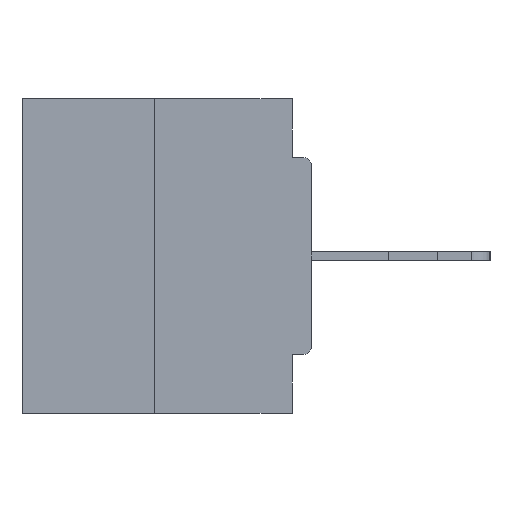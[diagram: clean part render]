
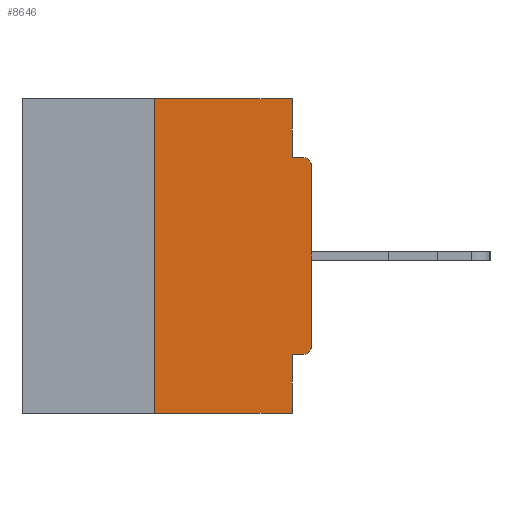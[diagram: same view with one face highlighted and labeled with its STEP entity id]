
A CAD part, left-side view. The second image highlights one B-rep face of the part: STEP entity #8646.
In plain terms, the highlighted planar face has unit normal (-1, 0, 0).
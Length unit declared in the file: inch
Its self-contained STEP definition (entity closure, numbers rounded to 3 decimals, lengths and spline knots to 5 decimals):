
#149 = ORIENTED_EDGE ( 'NONE', *, *, #8234, .F. ) ;
#605 = LINE ( 'NONE', #27355, #24808 ) ;
#615 = LINE ( 'NONE', #12109, #26705 ) ;
#1014 = EDGE_CURVE ( 'NONE', #3477, #11156, #14112, .T. ) ;
#1079 = VERTEX_POINT ( 'NONE', #6250 ) ;
#1119 = EDGE_CURVE ( 'NONE', #1079, #21119, #18806, .T. ) ;
#1353 = VERTEX_POINT ( 'NONE', #11446 ) ;
#1590 = DIRECTION ( 'NONE',  ( 0., 0., -1. ) ) ;
#3269 = CARTESIAN_POINT ( 'NONE',  ( 0., 0.031, 0. ) ) ;
#3477 = VERTEX_POINT ( 'NONE', #12547 ) ;
#3612 = ORIENTED_EDGE ( 'NONE', *, *, #9767, .F. ) ;
#3628 = CARTESIAN_POINT ( 'NONE',  ( 0., 0.015, -0.3915 ) ) ;
#3870 = CARTESIAN_POINT ( 'NONE',  ( 0., 0.031, -0.0935 ) ) ;
#4341 = ORIENTED_EDGE ( 'NONE', *, *, #8951, .T. ) ;
#4351 = ORIENTED_EDGE ( 'NONE', *, *, #15513, .F. ) ;
#4420 = VECTOR ( 'NONE', #23485, 39.37008 ) ;
#4448 = ORIENTED_EDGE ( 'NONE', *, *, #9944, .F. ) ;
#4817 = CARTESIAN_POINT ( 'NONE',  ( 0., 0.25, 0. ) ) ;
#4937 = DIRECTION ( 'NONE',  ( 0., -1., 0. ) ) ;
#5489 = PLANE ( 'NONE',  #23895 ) ;
#6250 = CARTESIAN_POINT ( 'NONE',  ( 0., 0.015, -0.4065 ) ) ;
#6367 = AXIS2_PLACEMENT_3D ( 'NONE', #28479, #19087, #1590 ) ;
#7471 = VERTEX_POINT ( 'NONE', #18476 ) ;
#8234 = EDGE_CURVE ( 'NONE', #21190, #18710, #13362, .T. ) ;
#8646 = ADVANCED_FACE ( 'NONE', ( #23142 ), #5489, .F. ) ;
#8951 = EDGE_CURVE ( 'NONE', #3477, #7471, #615, .T. ) ;
#9069 = CARTESIAN_POINT ( 'NONE',  ( 0., 0.015, -0.0935 ) ) ;
#9613 = VECTOR ( 'NONE', #9849, 39.37008 ) ;
#9767 = EDGE_CURVE ( 'NONE', #1079, #1353, #605, .T. ) ;
#9849 = DIRECTION ( 'NONE',  ( 0., -1., 0. ) ) ;
#9944 = EDGE_CURVE ( 'NONE', #1353, #7471, #24639, .T. ) ;
#9987 = DIRECTION ( 'NONE',  ( 0., 0., -1. ) ) ;
#10577 = CARTESIAN_POINT ( 'NONE',  ( 0., 0., 0. ) ) ;
#11148 = ORIENTED_EDGE ( 'NONE', *, *, #14624, .F. ) ;
#11156 = VERTEX_POINT ( 'NONE', #23710 ) ;
#11260 = DIRECTION ( 'NONE',  ( 0., 1., 0. ) ) ;
#11446 = CARTESIAN_POINT ( 'NONE',  ( 0., 0.031, -0.4065 ) ) ;
#12109 = CARTESIAN_POINT ( 'NONE',  ( 0., 0.46, -0.5 ) ) ;
#12180 = ORIENTED_EDGE ( 'NONE', *, *, #1014, .F. ) ;
#12547 = CARTESIAN_POINT ( 'NONE',  ( 0., 0.25, -0.5 ) ) ;
#13362 = LINE ( 'NONE', #24346, #19172 ) ;
#13501 = DIRECTION ( 'NONE',  ( 0., 0., -1. ) ) ;
#13649 = LINE ( 'NONE', #27414, #9613 ) ;
#14112 = LINE ( 'NONE', #4817, #4420 ) ;
#14342 = EDGE_CURVE ( 'NONE', #26387, #20639, #28772, .T. ) ;
#14620 = AXIS2_PLACEMENT_3D ( 'NONE', #3628, #28487, #23939 ) ;
#14624 = EDGE_CURVE ( 'NONE', #11156, #21190, #13649, .T. ) ;
#15513 = EDGE_CURVE ( 'NONE', #18710, #20639, #16740, .T. ) ;
#16740 = LINE ( 'NONE', #25235, #20365 ) ;
#16809 = EDGE_CURVE ( 'NONE', #21119, #26387, #26370, .T. ) ;
#17094 = VECTOR ( 'NONE', #24431, 39.37008 ) ;
#18476 = CARTESIAN_POINT ( 'NONE',  ( 0., 0.031, -0.5 ) ) ;
#18710 = VERTEX_POINT ( 'NONE', #3870 ) ;
#18806 = CIRCLE ( 'NONE', #14620, 0.015 ) ;
#19087 = DIRECTION ( 'NONE',  ( -1., 0., 0. ) ) ;
#19172 = VECTOR ( 'NONE', #13501, 39.37008 ) ;
#20365 = VECTOR ( 'NONE', #4937, 39.37008 ) ;
#20639 = VERTEX_POINT ( 'NONE', #9069 ) ;
#21119 = VERTEX_POINT ( 'NONE', #26602 ) ;
#21190 = VERTEX_POINT ( 'NONE', #3269 ) ;
#21809 = ORIENTED_EDGE ( 'NONE', *, *, #14342, .T. ) ;
#21879 = ORIENTED_EDGE ( 'NONE', *, *, #16809, .T. ) ;
#22956 = DIRECTION ( 'NONE',  ( 0., -1., 0. ) ) ;
#23142 = FACE_OUTER_BOUND ( 'NONE', #24683, .T. ) ;
#23287 = DIRECTION ( 'NONE',  ( 1., 0., 0. ) ) ;
#23485 = DIRECTION ( 'NONE',  ( 0., 0., 1. ) ) ;
#23710 = CARTESIAN_POINT ( 'NONE',  ( 0., 0.25, 0. ) ) ;
#23895 = AXIS2_PLACEMENT_3D ( 'NONE', #25642, #23287, #9987 ) ;
#23939 = DIRECTION ( 'NONE',  ( 0., 0., -1. ) ) ;
#24284 = CARTESIAN_POINT ( 'NONE',  ( 0., 0., -0.1085 ) ) ;
#24346 = CARTESIAN_POINT ( 'NONE',  ( 0., 0.031, 0. ) ) ;
#24431 = DIRECTION ( 'NONE',  ( 0., 0., 1. ) ) ;
#24639 = LINE ( 'NONE', #26475, #25735 ) ;
#24683 = EDGE_LOOP ( 'NONE', ( #11148, #12180, #4341, #4448, #3612, #26940, #21879, #21809, #4351, #149 ) ) ;
#24808 = VECTOR ( 'NONE', #11260, 39.37008 ) ;
#25235 = CARTESIAN_POINT ( 'NONE',  ( 0., 0., -0.0935 ) ) ;
#25642 = CARTESIAN_POINT ( 'NONE',  ( 0., 0.46, 0. ) ) ;
#25735 = VECTOR ( 'NONE', #26702, 39.37008 ) ;
#26370 = LINE ( 'NONE', #10577, #17094 ) ;
#26387 = VERTEX_POINT ( 'NONE', #24284 ) ;
#26475 = CARTESIAN_POINT ( 'NONE',  ( 0., 0.031, -0.5 ) ) ;
#26602 = CARTESIAN_POINT ( 'NONE',  ( 0., 0., -0.3915 ) ) ;
#26702 = DIRECTION ( 'NONE',  ( 0., 0., -1. ) ) ;
#26705 = VECTOR ( 'NONE', #22956, 39.37008 ) ;
#26940 = ORIENTED_EDGE ( 'NONE', *, *, #1119, .T. ) ;
#27355 = CARTESIAN_POINT ( 'NONE',  ( 0., 0., -0.4065 ) ) ;
#27414 = CARTESIAN_POINT ( 'NONE',  ( 0., 0.46, 0. ) ) ;
#28479 = CARTESIAN_POINT ( 'NONE',  ( 0., 0.015, -0.1085 ) ) ;
#28487 = DIRECTION ( 'NONE',  ( -1., 0., 0. ) ) ;
#28772 = CIRCLE ( 'NONE', #6367, 0.015 ) ;
